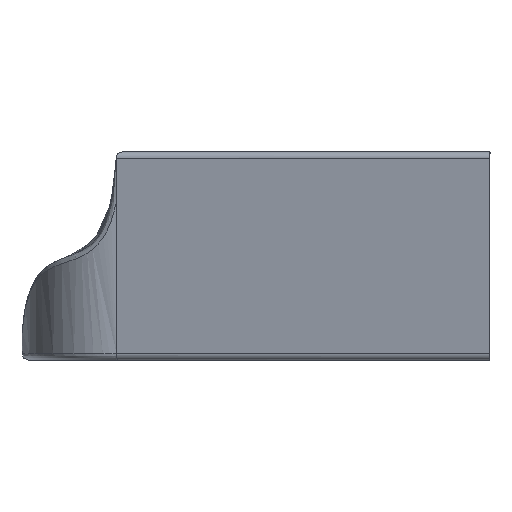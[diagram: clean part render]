
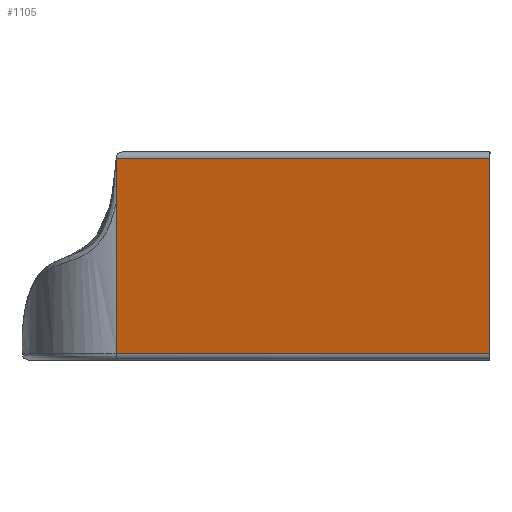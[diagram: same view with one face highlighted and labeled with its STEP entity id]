
A CAD part, left-side view. The second image highlights one B-rep face of the part: STEP entity #1105.
In plain terms, the highlighted planar face has unit normal (-0.966, 0.259, 0).
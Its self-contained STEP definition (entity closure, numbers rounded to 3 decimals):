
#30 = ORIENTED_EDGE ( 'NONE', *, *, #561, .T. ) ;
#49 = CARTESIAN_POINT ( 'NONE',  ( -13.295, 3.563, -7.75 ) ) ;
#93 = CARTESIAN_POINT ( 'NONE',  ( -22.178, -29.587, 8.25 ) ) ;
#115 = CARTESIAN_POINT ( 'NONE',  ( -14.25, 0., 4.313 ) ) ;
#143 = CARTESIAN_POINT ( 'NONE',  ( -14.25, 0., -7.75 ) ) ;
#335 = VERTEX_POINT ( 'NONE', #115 ) ;
#352 = CARTESIAN_POINT ( 'NONE',  ( -22.178, -29.587, 7.75 ) ) ;
#412 = DIRECTION ( 'NONE',  ( -0.259, -0.966, 0. ) ) ;
#414 = LINE ( 'NONE', #643, #960 ) ;
#426 = CARTESIAN_POINT ( 'NONE',  ( -14.25, 0., 7.75 ) ) ;
#561 = EDGE_CURVE ( 'NONE', #1009, #629, #574, .T. ) ;
#574 = LINE ( 'NONE', #426, #1443 ) ;
#615 = ORIENTED_EDGE ( 'NONE', *, *, #641, .F. ) ;
#629 = VERTEX_POINT ( 'NONE', #1211 ) ;
#641 = EDGE_CURVE ( 'NONE', #1009, #764, #835, .T. ) ;
#643 = CARTESIAN_POINT ( 'NONE',  ( -14.25, 0., -8.25 ) ) ;
#659 = DIRECTION ( 'NONE',  ( 0., 0., -1. ) ) ;
#673 = DIRECTION ( 'NONE',  ( 0., 0., -1. ) ) ;
#736 = LINE ( 'NONE', #995, #988 ) ;
#756 = DIRECTION ( 'NONE',  ( 0.259, 0.966, 0. ) ) ;
#757 = LINE ( 'NONE', #49, #1003 ) ;
#764 = VERTEX_POINT ( 'NONE', #1104 ) ;
#774 = EDGE_CURVE ( 'NONE', #629, #335, #736, .T. ) ;
#790 = VECTOR ( 'NONE', #659, 1000. ) ;
#802 = ORIENTED_EDGE ( 'NONE', *, *, #880, .T. ) ;
#835 = LINE ( 'NONE', #93, #790 ) ;
#846 = ORIENTED_EDGE ( 'NONE', *, *, #1421, .T. ) ;
#880 = EDGE_CURVE ( 'NONE', #335, #1242, #414, .T. ) ;
#909 = DIRECTION ( 'NONE',  ( 0.966, -0.259, 0. ) ) ;
#960 = VECTOR ( 'NONE', #1432, 1000. ) ;
#988 = VECTOR ( 'NONE', #673, 1000. ) ;
#995 = CARTESIAN_POINT ( 'NONE',  ( -14.25, 0., 8.25 ) ) ;
#1003 = VECTOR ( 'NONE', #412, 1000. ) ;
#1009 = VERTEX_POINT ( 'NONE', #352 ) ;
#1104 = CARTESIAN_POINT ( 'NONE',  ( -22.178, -29.587, -7.75 ) ) ;
#1105 = ADVANCED_FACE ( 'NONE', ( #1107 ), #1245, .F. ) ;
#1107 = FACE_OUTER_BOUND ( 'NONE', #1334, .T. ) ;
#1129 = CARTESIAN_POINT ( 'NONE',  ( -13.295, 3.563, 8.25 ) ) ;
#1211 = CARTESIAN_POINT ( 'NONE',  ( -14.25, 0., 7.75 ) ) ;
#1242 = VERTEX_POINT ( 'NONE', #143 ) ;
#1245 = PLANE ( 'NONE',  #1366 ) ;
#1284 = ORIENTED_EDGE ( 'NONE', *, *, #774, .T. ) ;
#1334 = EDGE_LOOP ( 'NONE', ( #615, #30, #1284, #802, #846 ) ) ;
#1366 = AXIS2_PLACEMENT_3D ( 'NONE', #1129, #909, #1369 ) ;
#1369 = DIRECTION ( 'NONE',  ( 0.259, 0.966, 0. ) ) ;
#1421 = EDGE_CURVE ( 'NONE', #1242, #764, #757, .T. ) ;
#1432 = DIRECTION ( 'NONE',  ( 0., 0., -1. ) ) ;
#1443 = VECTOR ( 'NONE', #756, 1000. ) ;
